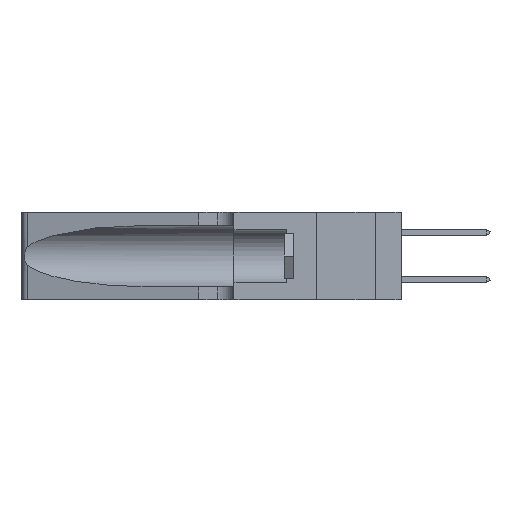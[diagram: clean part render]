
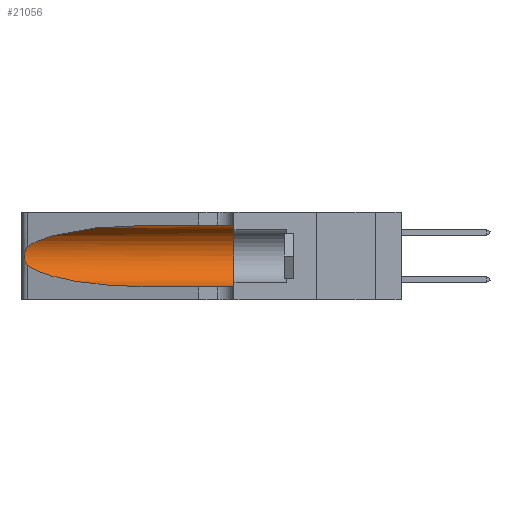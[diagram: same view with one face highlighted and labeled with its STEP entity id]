
A CAD part, left-side view. The second image highlights one B-rep face of the part: STEP entity #21056.
In plain terms, the highlighted cylindrical face has radius 3.308 mm (diameter 6.617 mm), a partial arc.
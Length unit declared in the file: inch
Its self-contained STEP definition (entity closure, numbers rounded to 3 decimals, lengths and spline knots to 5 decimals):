
#163 = ORIENTED_EDGE ( 'NONE', *, *, #326, .T. ) ;
#326 = EDGE_CURVE ( 'NONE', #7138, #30644, #13436, .T. ) ;
#781 = CARTESIAN_POINT ( 'NONE',  ( 0.26075, 1.23896, 0.178 ) ) ;
#1311 = VERTEX_POINT ( 'NONE', #13607 ) ;
#1608 = CIRCLE ( 'NONE', #26986, 0.13025 ) ;
#1988 = LINE ( 'NONE', #24850, #16365 ) ;
#2154 = EDGE_CURVE ( 'NONE', #8568, #30644, #1608, .T. ) ;
#3095 = CARTESIAN_POINT ( 'NONE',  ( 0.1305, 0.35, 0.05475 ) ) ;
#3818 = CARTESIAN_POINT ( 'NONE',  ( 0.25487, 1.22718, 0.14631 ) ) ;
#4955 = ORIENTED_EDGE ( 'NONE', *, *, #2154, .F. ) ;
#4979 = CARTESIAN_POINT ( 'NONE',  ( 0.26018, 1.23835, 0.19895 ) ) ;
#6807 = DIRECTION ( 'NONE',  ( 0., 1., 0. ) ) ;
#6829 = CARTESIAN_POINT ( 'NONE',  ( 0.2373, 1.15595, 0.28018 ) ) ;
#6911 = CYLINDRICAL_SURFACE ( 'NONE', #8282, 0.13025 ) ;
#7138 = VERTEX_POINT ( 'NONE', #20178 ) ;
#7477 = EDGE_CURVE ( 'NONE', #11684, #22306, #18542, .T. ) ;
#7873 = CARTESIAN_POINT ( 'NONE',  ( 0.25856, 1.23593, 0.16098 ) ) ;
#7913 = ORIENTED_EDGE ( 'NONE', *, *, #9070, .T. ) ;
#7970 = DIRECTION ( 'NONE',  ( 0., -1., 0. ) ) ;
#8061 = CARTESIAN_POINT ( 'NONE',  ( 0.1305, 1.61858, 0.05475 ) ) ;
#8143 = CARTESIAN_POINT ( 'NONE',  ( 0.25487, 1.22718, 0.22369 ) ) ;
#8282 = AXIS2_PLACEMENT_3D ( 'NONE', #29620, #24825, #15133 ) ;
#8398 = CARTESIAN_POINT ( 'NONE',  ( 0.1305, 0.72297, 0.05475 ) ) ;
#8568 = VERTEX_POINT ( 'NONE', #18002 ) ;
#8735 = CARTESIAN_POINT ( 'NONE',  ( 0.18966, 0.96281, 0.05475 ) ) ;
#9053 = DIRECTION ( 'NONE',  ( 0., 0., 1. ) ) ;
#9070 = EDGE_CURVE ( 'NONE', #22306, #1311, #23822, .T. ) ;
#10582 = ORIENTED_EDGE ( 'NONE', *, *, #14736, .F. ) ;
#11157 = CARTESIAN_POINT ( 'NONE',  ( 0.25555, 1.22993, 0.14849 ) ) ;
#11507 = CARTESIAN_POINT ( 'NONE',  ( 0.26017, 1.23833, 0.17102 ) ) ;
#11684 = VERTEX_POINT ( 'NONE', #20999 ) ;
#12428 = CARTESIAN_POINT ( 'NONE',  ( 0.25487, 1.22718, 0.22369 ) ) ;
#13061 = DIRECTION ( 'NONE',  ( 0., -1., 0. ) ) ;
#13436 = LINE ( 'NONE', #8061, #18311 ) ;
#13607 = CARTESIAN_POINT ( 'NONE',  ( 0.25487, 1.22718, 0.14631 ) ) ;
#14736 = EDGE_CURVE ( 'NONE', #11684, #8568, #1988, .T. ) ;
#14823 =( BOUNDED_CURVE ( )  B_SPLINE_CURVE ( 3, ( #3818, #22880, #8735, #8398 ),
 .UNSPECIFIED., .F., .T. ) 
 B_SPLINE_CURVE_WITH_KNOTS ( ( 4, 4 ),
 ( 3.44316, 4.71239 ),
 .UNSPECIFIED. ) 
 CURVE ( )  GEOMETRIC_REPRESENTATION_ITEM ( )  RATIONAL_B_SPLINE_CURVE ( ( 1., 0.87, 0.87, 1. ) ) 
 REPRESENTATION_ITEM ( '' )  );
#15133 = DIRECTION ( 'NONE',  ( 0., 0., -1. ) ) ;
#15469 = CARTESIAN_POINT ( 'NONE',  ( 0.25787, 1.23484, 0.2124 ) ) ;
#15892 = CARTESIAN_POINT ( 'NONE',  ( 0.25639, 1.23186, 0.15144 ) ) ;
#16365 = VECTOR ( 'NONE', #7970, 39.37008 ) ;
#16764 = CARTESIAN_POINT ( 'NONE',  ( 0.1305, 0.72297, 0.31525 ) ) ;
#17447 = FACE_OUTER_BOUND ( 'NONE', #21301, .T. ) ;
#18002 = CARTESIAN_POINT ( 'NONE',  ( 0.1305, 0.35, 0.31525 ) ) ;
#18311 = VECTOR ( 'NONE', #13061, 39.37008 ) ;
#18542 =( BOUNDED_CURVE ( )  B_SPLINE_CURVE ( 3, ( #16764, #26082, #6829, #18969 ),
 .UNSPECIFIED., .F., .T. ) 
 B_SPLINE_CURVE_WITH_KNOTS ( ( 4, 4 ),
 ( 1.5708, 2.84003 ),
 .UNSPECIFIED. ) 
 CURVE ( )  GEOMETRIC_REPRESENTATION_ITEM ( )  RATIONAL_B_SPLINE_CURVE ( ( 1., 0.87, 0.87, 1. ) ) 
 REPRESENTATION_ITEM ( '' )  );
#18969 = CARTESIAN_POINT ( 'NONE',  ( 0.25487, 1.22718, 0.22369 ) ) ;
#20178 = CARTESIAN_POINT ( 'NONE',  ( 0.1305, 0.72297, 0.05475 ) ) ;
#20999 = CARTESIAN_POINT ( 'NONE',  ( 0.1305, 0.72297, 0.31525 ) ) ;
#21056 = ADVANCED_FACE ( 'NONE', ( #17447 ), #6911, .F. ) ;
#21301 = EDGE_LOOP ( 'NONE', ( #21844, #7913, #26352, #163, #4955, #10582 ) ) ;
#21844 = ORIENTED_EDGE ( 'NONE', *, *, #7477, .T. ) ;
#21864 = EDGE_CURVE ( 'NONE', #1311, #7138, #14823, .T. ) ;
#22306 = VERTEX_POINT ( 'NONE', #8143 ) ;
#22880 = CARTESIAN_POINT ( 'NONE',  ( 0.2373, 1.15595, 0.08982 ) ) ;
#22930 = CARTESIAN_POINT ( 'NONE',  ( 0.25854, 1.2359, 0.20912 ) ) ;
#23555 = CARTESIAN_POINT ( 'NONE',  ( 0.1305, 0.35, 0.185 ) ) ;
#23822 = B_SPLINE_CURVE_WITH_KNOTS ( 'NONE', 3,
 ( #12428, #24724, #27293, #15469, #22930, #4979, #26595, #781, #11507, #7873, #28046, #15892, #11157, #30580 ),
 .UNSPECIFIED., .F., .F.,
 ( 4, 2, 2, 2, 2, 2, 4 ),
 ( 0., 0.00027, 0.00053, 0.00107, 0.0016, 0.00187, 0.00214 ),
 .UNSPECIFIED. ) ;
#24724 = CARTESIAN_POINT ( 'NONE',  ( 0.25555, 1.22994, 0.2215 ) ) ;
#24825 = DIRECTION ( 'NONE',  ( 0., -1., 0. ) ) ;
#24850 = CARTESIAN_POINT ( 'NONE',  ( 0.1305, 1.61858, 0.31525 ) ) ;
#26082 = CARTESIAN_POINT ( 'NONE',  ( 0.18966, 0.96281, 0.31525 ) ) ;
#26352 = ORIENTED_EDGE ( 'NONE', *, *, #21864, .T. ) ;
#26595 = CARTESIAN_POINT ( 'NONE',  ( 0.26075, 1.23896, 0.19203 ) ) ;
#26986 = AXIS2_PLACEMENT_3D ( 'NONE', #23555, #6807, #9053 ) ;
#27293 = CARTESIAN_POINT ( 'NONE',  ( 0.25639, 1.23184, 0.21858 ) ) ;
#28046 = CARTESIAN_POINT ( 'NONE',  ( 0.25789, 1.23486, 0.15765 ) ) ;
#29620 = CARTESIAN_POINT ( 'NONE',  ( 0.1305, 1.61858, 0.185 ) ) ;
#30580 = CARTESIAN_POINT ( 'NONE',  ( 0.25487, 1.22718, 0.14631 ) ) ;
#30644 = VERTEX_POINT ( 'NONE', #3095 ) ;
